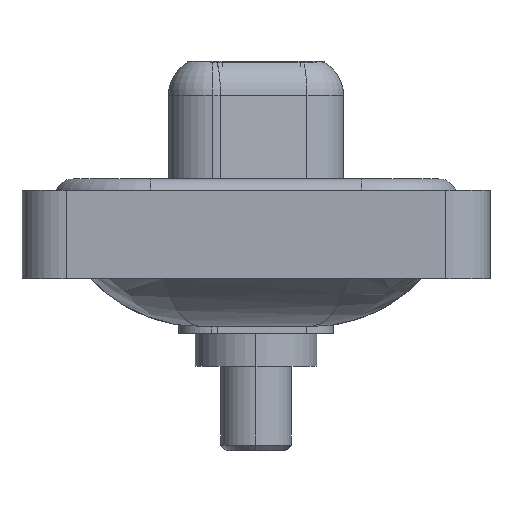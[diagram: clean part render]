
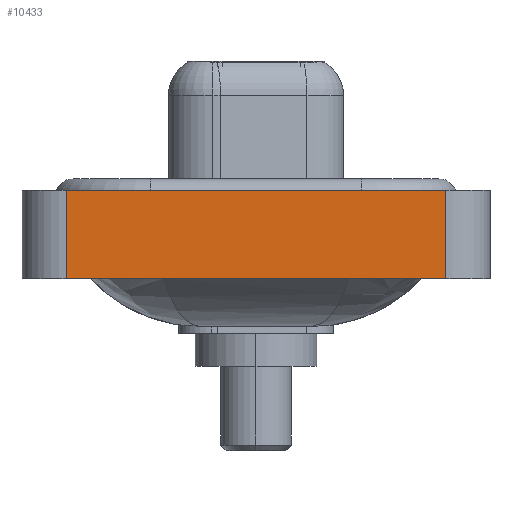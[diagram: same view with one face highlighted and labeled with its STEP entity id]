
A CAD part, left-side view. The second image highlights one B-rep face of the part: STEP entity #10433.
In plain terms, the highlighted planar face has unit normal (-1, 0, 0).
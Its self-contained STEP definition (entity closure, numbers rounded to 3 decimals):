
#413 = CARTESIAN_POINT ( 'NONE',  ( -7.35, -8.55, 0.4 ) ) ;
#541 = ORIENTED_EDGE ( 'NONE', *, *, #9491, .T. ) ;
#597 = ORIENTED_EDGE ( 'NONE', *, *, #754, .F. ) ;
#625 = DIRECTION ( 'NONE',  ( 0., -1., 0. ) ) ;
#754 = EDGE_CURVE ( 'NONE', #14172, #9644, #10888, .T. ) ;
#864 = VECTOR ( 'NONE', #4348, 1000. ) ;
#890 = VERTEX_POINT ( 'NONE', #10270 ) ;
#1697 = EDGE_CURVE ( 'NONE', #14172, #890, #12316, .T. ) ;
#1882 = DIRECTION ( 'NONE',  ( -1., 0., 0. ) ) ;
#2781 = AXIS2_PLACEMENT_3D ( 'NONE', #8290, #1882, #7019 ) ;
#4315 = CARTESIAN_POINT ( 'NONE',  ( -7.35, 8.55, 0.4 ) ) ;
#4348 = DIRECTION ( 'NONE',  ( 0., 0., 1. ) ) ;
#6812 = CARTESIAN_POINT ( 'NONE',  ( -7.35, 8.55, -3.6 ) ) ;
#7019 = DIRECTION ( 'NONE',  ( 0., 0., 1. ) ) ;
#7056 = ORIENTED_EDGE ( 'NONE', *, *, #14598, .F. ) ;
#7193 = DIRECTION ( 'NONE',  ( 0., 0., 1. ) ) ;
#7548 = VERTEX_POINT ( 'NONE', #413 ) ;
#7717 = VECTOR ( 'NONE', #13421, 1000. ) ;
#8290 = CARTESIAN_POINT ( 'NONE',  ( -7.35, -8.55, -3.6 ) ) ;
#8522 = VECTOR ( 'NONE', #7193, 1000. ) ;
#9317 = CARTESIAN_POINT ( 'NONE',  ( -7.35, -8.55, 0.4 ) ) ;
#9491 = EDGE_CURVE ( 'NONE', #890, #7548, #14601, .T. ) ;
#9644 = VERTEX_POINT ( 'NONE', #4315 ) ;
#10270 = CARTESIAN_POINT ( 'NONE',  ( -7.35, -8.55, -3.6 ) ) ;
#10433 = ADVANCED_FACE ( 'NONE', ( #10797 ), #15937, .T. ) ;
#10510 = EDGE_LOOP ( 'NONE', ( #541, #7056, #597, #15032 ) ) ;
#10797 = FACE_OUTER_BOUND ( 'NONE', #10510, .T. ) ;
#10888 = LINE ( 'NONE', #10973, #8522 ) ;
#10893 = CARTESIAN_POINT ( 'NONE',  ( -7.35, -8.55, -3.6 ) ) ;
#10973 = CARTESIAN_POINT ( 'NONE',  ( -7.35, 8.55, -3.6 ) ) ;
#12316 = LINE ( 'NONE', #10893, #13399 ) ;
#13399 = VECTOR ( 'NONE', #625, 1000. ) ;
#13421 = DIRECTION ( 'NONE',  ( 0., -1., 0. ) ) ;
#14172 = VERTEX_POINT ( 'NONE', #6812 ) ;
#14598 = EDGE_CURVE ( 'NONE', #9644, #7548, #14935, .T. ) ;
#14601 = LINE ( 'NONE', #15870, #864 ) ;
#14935 = LINE ( 'NONE', #9317, #7717 ) ;
#15032 = ORIENTED_EDGE ( 'NONE', *, *, #1697, .T. ) ;
#15870 = CARTESIAN_POINT ( 'NONE',  ( -7.35, -8.55, -3.6 ) ) ;
#15937 = PLANE ( 'NONE',  #2781 ) ;
